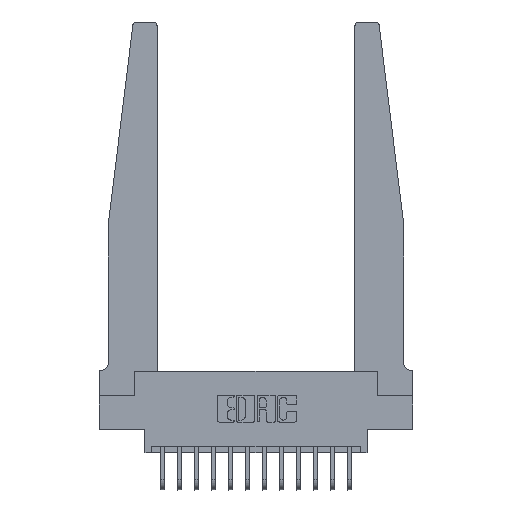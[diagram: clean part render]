
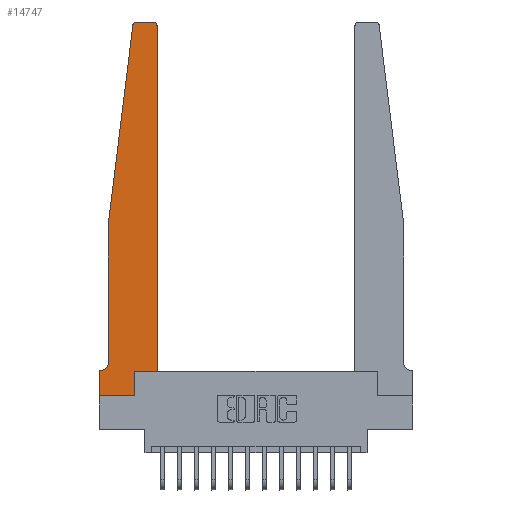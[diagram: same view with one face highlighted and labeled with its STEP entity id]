
A CAD part, top view. The second image highlights one B-rep face of the part: STEP entity #14747.
In plain terms, the highlighted planar face has unit normal (0, 0, 1).
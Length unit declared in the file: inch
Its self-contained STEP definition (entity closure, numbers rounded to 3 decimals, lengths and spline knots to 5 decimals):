
#100 = VERTEX_POINT ( 'NONE', #1005 ) ;
#135 = VERTEX_POINT ( 'NONE', #9101 ) ;
#525 = AXIS2_PLACEMENT_3D ( 'NONE', #4903, #13829, #6184 ) ;
#590 = ORIENTED_EDGE ( 'NONE', *, *, #645, .T. ) ;
#645 = EDGE_CURVE ( 'NONE', #14093, #9913, #10650, .T. ) ;
#852 = EDGE_CURVE ( 'NONE', #9663, #6649, #14593, .T. ) ;
#1005 = CARTESIAN_POINT ( 'NONE',  ( 0.425, 0.18, 0.37 ) ) ;
#1091 = CARTESIAN_POINT ( 'NONE',  ( 0.2605, 0.18, 0.37 ) ) ;
#1159 = DIRECTION ( 'NONE',  ( 0., 0., 1. ) ) ;
#1776 = ORIENTED_EDGE ( 'NONE', *, *, #852, .T. ) ;
#1930 = VERTEX_POINT ( 'NONE', #15472 ) ;
#2264 = EDGE_CURVE ( 'NONE', #15068, #5294, #11185, .T. ) ;
#2537 = ORIENTED_EDGE ( 'NONE', *, *, #11573, .T. ) ;
#2574 = DIRECTION ( 'NONE',  ( 0., 1., 0. ) ) ;
#2609 = VECTOR ( 'NONE', #13919, 39.37008 ) ;
#2781 = CIRCLE ( 'NONE', #13590, 0.05 ) ;
#3012 = LINE ( 'NONE', #16386, #2609 ) ;
#3113 = LINE ( 'NONE', #9502, #6524 ) ;
#3316 = EDGE_CURVE ( 'NONE', #135, #9663, #11604, .T. ) ;
#3625 = VERTEX_POINT ( 'NONE', #8043 ) ;
#3867 = VECTOR ( 'NONE', #13867, 39.37008 ) ;
#4457 = VECTOR ( 'NONE', #4615, 39.37008 ) ;
#4615 = DIRECTION ( 'NONE',  ( -1., 0., 0. ) ) ;
#4765 = CARTESIAN_POINT ( 'NONE',  ( 0.065, 1.25, 0.37 ) ) ;
#4903 = CARTESIAN_POINT ( 'NONE',  ( 0.27653, 2.72, 0.37 ) ) ;
#4990 = DIRECTION ( 'NONE',  ( 0., 1., 0. ) ) ;
#5049 = EDGE_CURVE ( 'NONE', #3625, #1930, #2781, .T. ) ;
#5096 = CARTESIAN_POINT ( 'NONE',  ( 0.25, 2.75, 0.37 ) ) ;
#5266 = ORIENTED_EDGE ( 'NONE', *, *, #3316, .T. ) ;
#5282 = LINE ( 'NONE', #8090, #11671 ) ;
#5294 = VERTEX_POINT ( 'NONE', #6520 ) ;
#6184 = DIRECTION ( 'NONE',  ( 1., 0., 0. ) ) ;
#6457 = ORIENTED_EDGE ( 'NONE', *, *, #13106, .T. ) ;
#6472 = DIRECTION ( 'NONE',  ( 1., 0., 0. ) ) ;
#6514 = LINE ( 'NONE', #14099, #6908 ) ;
#6520 = CARTESIAN_POINT ( 'NONE',  ( 0.2605, 0.18, 0.37 ) ) ;
#6524 = VECTOR ( 'NONE', #6986, 39.37008 ) ;
#6546 = AXIS2_PLACEMENT_3D ( 'NONE', #8859, #1159, #10129 ) ;
#6628 = FACE_OUTER_BOUND ( 'NONE', #9854, .T. ) ;
#6649 = VERTEX_POINT ( 'NONE', #13601 ) ;
#6751 = EDGE_CURVE ( 'NONE', #6649, #14093, #8530, .T. ) ;
#6880 = EDGE_CURVE ( 'NONE', #5294, #100, #6514, .T. ) ;
#6908 = VECTOR ( 'NONE', #6472, 39.37008 ) ;
#6986 = DIRECTION ( 'NONE',  ( -1., 0., 0. ) ) ;
#7006 = ORIENTED_EDGE ( 'NONE', *, *, #16207, .T. ) ;
#7116 = CARTESIAN_POINT ( 'NONE',  ( 0.015, 0.2375, 0.37 ) ) ;
#7271 = DIRECTION ( 'NONE',  ( 0., 0., 1. ) ) ;
#8043 = CARTESIAN_POINT ( 'NONE',  ( 0.065, 0.2375, 0.37 ) ) ;
#8068 = CARTESIAN_POINT ( 'NONE',  ( 0., 0., 0.37 ) ) ;
#8082 = EDGE_CURVE ( 'NONE', #100, #135, #12667, .T. ) ;
#8090 = CARTESIAN_POINT ( 'NONE',  ( 0., 0., 0.37 ) ) ;
#8124 = ORIENTED_EDGE ( 'NONE', *, *, #6880, .T. ) ;
#8148 = ORIENTED_EDGE ( 'NONE', *, *, #15079, .T. ) ;
#8444 = DIRECTION ( 'NONE',  ( -1., 0., 0. ) ) ;
#8530 = CIRCLE ( 'NONE', #525, 0.03 ) ;
#8859 = CARTESIAN_POINT ( 'NONE',  ( 0., 0.1875, 0.37 ) ) ;
#9101 = CARTESIAN_POINT ( 'NONE',  ( 0.425, 2.72, 0.37 ) ) ;
#9354 = DIRECTION ( 'NONE',  ( 0., -1., 0. ) ) ;
#9502 = CARTESIAN_POINT ( 'NONE',  ( 0.065, 0.1875, 0.37 ) ) ;
#9663 = VERTEX_POINT ( 'NONE', #12919 ) ;
#9736 = ORIENTED_EDGE ( 'NONE', *, *, #8082, .T. ) ;
#9854 = EDGE_LOOP ( 'NONE', ( #1776, #11712, #590, #7006, #14327, #2537, #6457, #8148, #10993, #8124, #9736, #5266 ) ) ;
#9913 = VERTEX_POINT ( 'NONE', #4765 ) ;
#10129 = DIRECTION ( 'NONE',  ( 1., 0., 0. ) ) ;
#10650 = LINE ( 'NONE', #13971, #3867 ) ;
#10908 = AXIS2_PLACEMENT_3D ( 'NONE', #14879, #7271, #16122 ) ;
#10993 = ORIENTED_EDGE ( 'NONE', *, *, #2264, .T. ) ;
#11154 = CARTESIAN_POINT ( 'NONE',  ( 0.24675, 2.72367, 0.37 ) ) ;
#11185 = LINE ( 'NONE', #1091, #14183 ) ;
#11573 = EDGE_CURVE ( 'NONE', #1930, #15581, #3113, .T. ) ;
#11604 = CIRCLE ( 'NONE', #10908, 0.03 ) ;
#11671 = VECTOR ( 'NONE', #9354, 39.37008 ) ;
#11712 = ORIENTED_EDGE ( 'NONE', *, *, #6751, .T. ) ;
#12282 = CARTESIAN_POINT ( 'NONE',  ( 0., 0.1875, 0.37 ) ) ;
#12382 = CARTESIAN_POINT ( 'NONE',  ( 0.065, 1.25, 0.37 ) ) ;
#12651 = CARTESIAN_POINT ( 'NONE',  ( 0.2605, 0., 0.37 ) ) ;
#12667 = LINE ( 'NONE', #14073, #16345 ) ;
#12919 = CARTESIAN_POINT ( 'NONE',  ( 0.395, 2.75, 0.37 ) ) ;
#13106 = EDGE_CURVE ( 'NONE', #15581, #13765, #5282, .T. ) ;
#13361 = LINE ( 'NONE', #12382, #16248 ) ;
#13590 = AXIS2_PLACEMENT_3D ( 'NONE', #7116, #15968, #8444 ) ;
#13601 = CARTESIAN_POINT ( 'NONE',  ( 0.27653, 2.75, 0.37 ) ) ;
#13656 = DIRECTION ( 'NONE',  ( 0., -1., 0. ) ) ;
#13765 = VERTEX_POINT ( 'NONE', #8068 ) ;
#13829 = DIRECTION ( 'NONE',  ( 0., 0., 1. ) ) ;
#13867 = DIRECTION ( 'NONE',  ( -0.122, -0.992, 0. ) ) ;
#13919 = DIRECTION ( 'NONE',  ( 1., 0., 0. ) ) ;
#13971 = CARTESIAN_POINT ( 'NONE',  ( 0.065, 1.25, 0.37 ) ) ;
#14073 = CARTESIAN_POINT ( 'NONE',  ( 0.425, 0.18, 0.37 ) ) ;
#14093 = VERTEX_POINT ( 'NONE', #11154 ) ;
#14099 = CARTESIAN_POINT ( 'NONE',  ( 0.425, 0.18, 0.37 ) ) ;
#14183 = VECTOR ( 'NONE', #4990, 39.37008 ) ;
#14327 = ORIENTED_EDGE ( 'NONE', *, *, #5049, .T. ) ;
#14593 = LINE ( 'NONE', #5096, #4457 ) ;
#14747 = ADVANCED_FACE ( 'NONE', ( #6628 ), #15087, .T. ) ;
#14879 = CARTESIAN_POINT ( 'NONE',  ( 0.395, 2.72, 0.37 ) ) ;
#15068 = VERTEX_POINT ( 'NONE', #12651 ) ;
#15079 = EDGE_CURVE ( 'NONE', #13765, #15068, #3012, .T. ) ;
#15087 = PLANE ( 'NONE',  #6546 ) ;
#15472 = CARTESIAN_POINT ( 'NONE',  ( 0.015, 0.1875, 0.37 ) ) ;
#15581 = VERTEX_POINT ( 'NONE', #12282 ) ;
#15968 = DIRECTION ( 'NONE',  ( 0., 0., -1. ) ) ;
#16122 = DIRECTION ( 'NONE',  ( 1., 0., 0. ) ) ;
#16207 = EDGE_CURVE ( 'NONE', #9913, #3625, #13361, .T. ) ;
#16248 = VECTOR ( 'NONE', #13656, 39.37008 ) ;
#16345 = VECTOR ( 'NONE', #2574, 39.37008 ) ;
#16386 = CARTESIAN_POINT ( 'NONE',  ( 0., 0., 0.37 ) ) ;
